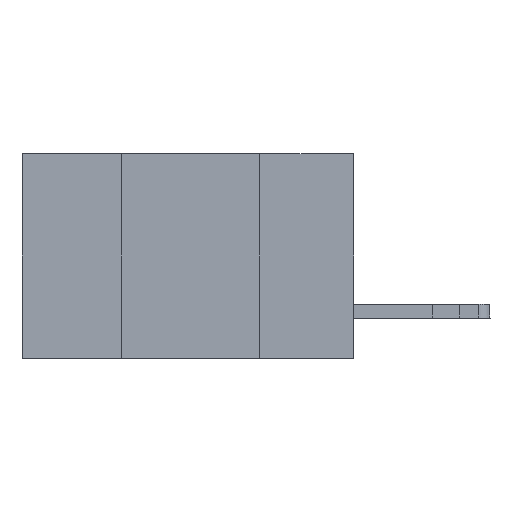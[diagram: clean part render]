
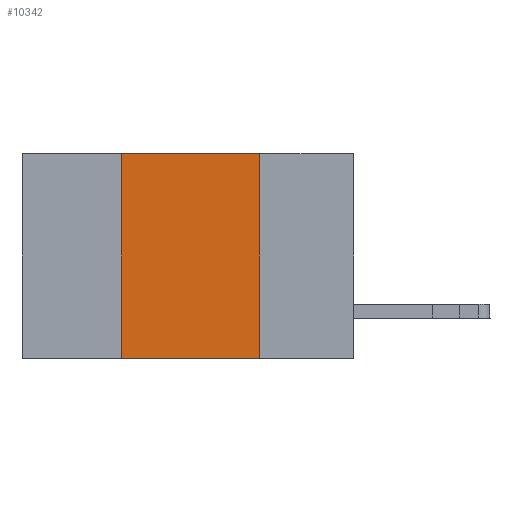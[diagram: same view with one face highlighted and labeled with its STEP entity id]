
A CAD part, left-side view. The second image highlights one B-rep face of the part: STEP entity #10342.
In plain terms, the highlighted planar face has unit normal (-1, 0, 0).
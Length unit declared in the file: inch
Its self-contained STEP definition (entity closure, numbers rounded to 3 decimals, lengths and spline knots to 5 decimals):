
#667 = CARTESIAN_POINT ( 'NONE',  ( 0., 0.17, -0.37 ) ) ;
#937 = DIRECTION ( 'NONE',  ( 0., -1., 0. ) ) ;
#1385 = PLANE ( 'NONE',  #2233 ) ;
#1529 = VECTOR ( 'NONE', #11340, 39.37008 ) ;
#1721 = CARTESIAN_POINT ( 'NONE',  ( 0., 0.17, 0. ) ) ;
#1831 = VECTOR ( 'NONE', #937, 39.37008 ) ;
#2233 = AXIS2_PLACEMENT_3D ( 'NONE', #6343, #17743, #7969 ) ;
#2643 = DIRECTION ( 'NONE',  ( 0., 0., -1. ) ) ;
#2694 = EDGE_CURVE ( 'NONE', #13094, #19601, #14037, .T. ) ;
#2804 = EDGE_LOOP ( 'NONE', ( #10432, #11981, #8873, #13219 ) ) ;
#2851 = EDGE_CURVE ( 'NONE', #13094, #4090, #19649, .T. ) ;
#3045 = VERTEX_POINT ( 'NONE', #1721 ) ;
#3821 = CARTESIAN_POINT ( 'NONE',  ( 0., 0.42, 0. ) ) ;
#4090 = VERTEX_POINT ( 'NONE', #667 ) ;
#6343 = CARTESIAN_POINT ( 'NONE',  ( 0., 0.6, 0. ) ) ;
#6555 = VECTOR ( 'NONE', #2643, 39.37008 ) ;
#7197 = LINE ( 'NONE', #20496, #1831 ) ;
#7969 = DIRECTION ( 'NONE',  ( 0., 0., -1. ) ) ;
#8099 = CARTESIAN_POINT ( 'NONE',  ( 0., 0.6, -0.37 ) ) ;
#8174 = DIRECTION ( 'NONE',  ( 0., -1., 0. ) ) ;
#8321 = CARTESIAN_POINT ( 'NONE',  ( 0., 0.42, -0.37 ) ) ;
#8873 = ORIENTED_EDGE ( 'NONE', *, *, #2694, .F. ) ;
#10342 = ADVANCED_FACE ( 'NONE', ( #14218 ), #1385, .F. ) ;
#10432 = ORIENTED_EDGE ( 'NONE', *, *, #21128, .F. ) ;
#11340 = DIRECTION ( 'NONE',  ( 0., 0., 1. ) ) ;
#11981 = ORIENTED_EDGE ( 'NONE', *, *, #12794, .F. ) ;
#12794 = EDGE_CURVE ( 'NONE', #19601, #3045, #7197, .T. ) ;
#13045 = CARTESIAN_POINT ( 'NONE',  ( 0., 0.42, 0. ) ) ;
#13094 = VERTEX_POINT ( 'NONE', #8321 ) ;
#13219 = ORIENTED_EDGE ( 'NONE', *, *, #2851, .T. ) ;
#13990 = CARTESIAN_POINT ( 'NONE',  ( 0., 0.17, 0. ) ) ;
#14037 = LINE ( 'NONE', #13045, #1529 ) ;
#14218 = FACE_OUTER_BOUND ( 'NONE', #2804, .T. ) ;
#15297 = VECTOR ( 'NONE', #8174, 39.37008 ) ;
#17743 = DIRECTION ( 'NONE',  ( 1., 0., 0. ) ) ;
#19550 = LINE ( 'NONE', #13990, #6555 ) ;
#19601 = VERTEX_POINT ( 'NONE', #3821 ) ;
#19649 = LINE ( 'NONE', #8099, #15297 ) ;
#20496 = CARTESIAN_POINT ( 'NONE',  ( 0., 0.6, 0. ) ) ;
#21128 = EDGE_CURVE ( 'NONE', #3045, #4090, #19550, .T. ) ;
